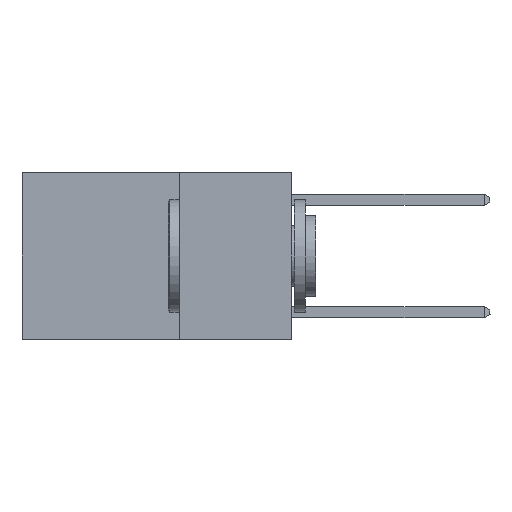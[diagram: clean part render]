
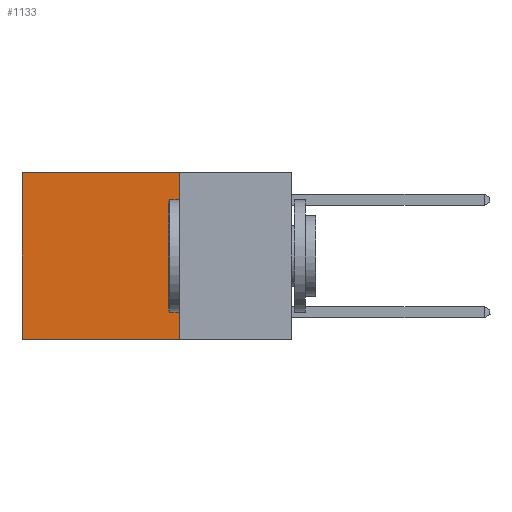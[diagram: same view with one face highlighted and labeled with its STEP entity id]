
A CAD part, left-side view. The second image highlights one B-rep face of the part: STEP entity #1133.
In plain terms, the highlighted planar face has unit normal (-1, 0, 0).
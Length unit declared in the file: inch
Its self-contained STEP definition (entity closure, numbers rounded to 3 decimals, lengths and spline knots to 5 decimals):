
#185 = CARTESIAN_POINT ( 'NONE',  ( 0.2625, 0.6, -0.37 ) ) ;
#498 = DIRECTION ( 'NONE',  ( 0., 1., 0. ) ) ;
#1037 = VECTOR ( 'NONE', #8347, 39.37008 ) ;
#1133 = ADVANCED_FACE ( 'NONE', ( #3720 ), #13193, .F. ) ;
#1632 = LINE ( 'NONE', #10904, #9509 ) ;
#2133 = CARTESIAN_POINT ( 'NONE',  ( 0.2625, 0.6, 0. ) ) ;
#2151 = ORIENTED_EDGE ( 'NONE', *, *, #13604, .T. ) ;
#2616 = VECTOR ( 'NONE', #14324, 39.37008 ) ;
#3151 = CARTESIAN_POINT ( 'NONE',  ( 0.2625, 0.25, -0.37 ) ) ;
#3484 = CARTESIAN_POINT ( 'NONE',  ( 0.2625, 0.25, 0. ) ) ;
#3720 = FACE_OUTER_BOUND ( 'NONE', #14392, .T. ) ;
#3964 = ORIENTED_EDGE ( 'NONE', *, *, #6608, .T. ) ;
#4092 = LINE ( 'NONE', #8509, #2616 ) ;
#4746 = VERTEX_POINT ( 'NONE', #185 ) ;
#6608 = EDGE_CURVE ( 'NONE', #14182, #4746, #4092, .T. ) ;
#7777 = VERTEX_POINT ( 'NONE', #12779 ) ;
#8285 = AXIS2_PLACEMENT_3D ( 'NONE', #9703, #14375, #14221 ) ;
#8347 = DIRECTION ( 'NONE',  ( 0., 0., -1. ) ) ;
#8509 = CARTESIAN_POINT ( 'NONE',  ( 0.2625, 0.6, 0. ) ) ;
#8657 = ORIENTED_EDGE ( 'NONE', *, *, #12991, .F. ) ;
#8678 = VERTEX_POINT ( 'NONE', #3484 ) ;
#8769 = DIRECTION ( 'NONE',  ( 0., 1., 0. ) ) ;
#9001 = LINE ( 'NONE', #3151, #12251 ) ;
#9509 = VECTOR ( 'NONE', #498, 39.37008 ) ;
#9703 = CARTESIAN_POINT ( 'NONE',  ( 0.2625, 0.25, 0. ) ) ;
#10846 = CARTESIAN_POINT ( 'NONE',  ( 0.2625, 0.25, 0. ) ) ;
#10904 = CARTESIAN_POINT ( 'NONE',  ( 0.2625, 0.25, 0. ) ) ;
#11621 = LINE ( 'NONE', #10846, #1037 ) ;
#12251 = VECTOR ( 'NONE', #8769, 39.37008 ) ;
#12779 = CARTESIAN_POINT ( 'NONE',  ( 0.2625, 0.25, -0.37 ) ) ;
#12991 = EDGE_CURVE ( 'NONE', #8678, #7777, #11621, .T. ) ;
#13193 = PLANE ( 'NONE',  #8285 ) ;
#13604 = EDGE_CURVE ( 'NONE', #8678, #14182, #1632, .T. ) ;
#14182 = VERTEX_POINT ( 'NONE', #2133 ) ;
#14221 = DIRECTION ( 'NONE',  ( 0., 0., -1. ) ) ;
#14324 = DIRECTION ( 'NONE',  ( 0., 0., -1. ) ) ;
#14375 = DIRECTION ( 'NONE',  ( 1., 0., 0. ) ) ;
#14392 = EDGE_LOOP ( 'NONE', ( #3964, #14842, #8657, #2151 ) ) ;
#14842 = ORIENTED_EDGE ( 'NONE', *, *, #14955, .F. ) ;
#14955 = EDGE_CURVE ( 'NONE', #7777, #4746, #9001, .T. ) ;
